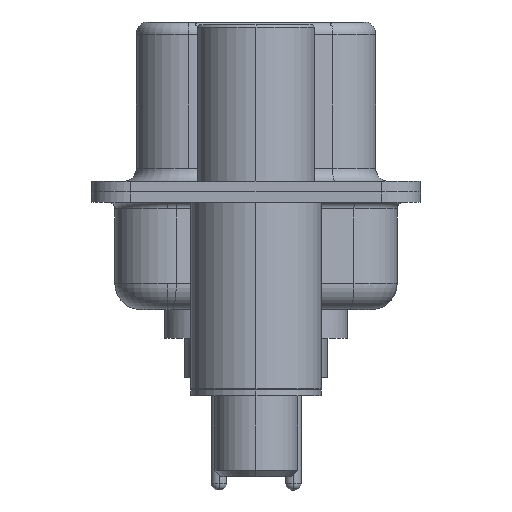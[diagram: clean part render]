
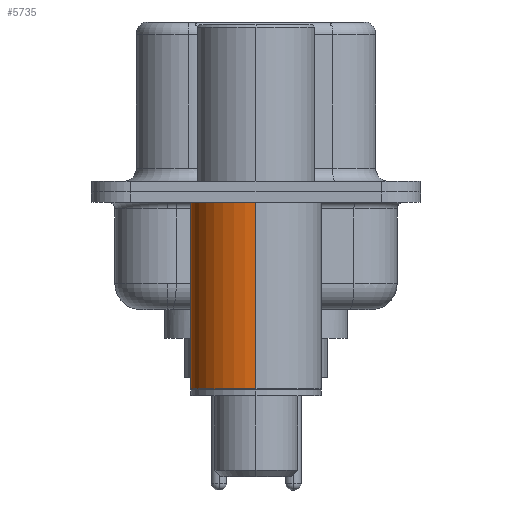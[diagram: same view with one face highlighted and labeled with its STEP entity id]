
A CAD part, left-side view. The second image highlights one B-rep face of the part: STEP entity #5735.
In plain terms, the highlighted cylindrical face has radius 2.5 mm (diameter 5 mm), a partial arc.
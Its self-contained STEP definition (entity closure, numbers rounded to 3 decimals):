
#570 = ORIENTED_EDGE ( 'NONE', *, *, #3838, .F. ) ;
#767 = CARTESIAN_POINT ( 'NONE',  ( 0., 0., -7.525 ) ) ;
#917 = EDGE_LOOP ( 'NONE', ( #12664, #6063, #570, #17866 ) ) ;
#1201 = AXIS2_PLACEMENT_3D ( 'NONE', #21291, #8077, #12361 ) ;
#1298 = VERTEX_POINT ( 'NONE', #20996 ) ;
#2603 = VECTOR ( 'NONE', #26259, 1000. ) ;
#3025 = DIRECTION ( 'NONE',  ( 1., 0., 0. ) ) ;
#3763 = CYLINDRICAL_SURFACE ( 'NONE', #17589, 2.5 ) ;
#3836 = VERTEX_POINT ( 'NONE', #18754 ) ;
#3838 = EDGE_CURVE ( 'NONE', #1298, #3836, #13167, .T. ) ;
#5735 = ADVANCED_FACE ( 'NONE', ( #10599 ), #3763, .T. ) ;
#6063 = ORIENTED_EDGE ( 'NONE', *, *, #20919, .T. ) ;
#8077 = DIRECTION ( 'NONE',  ( 0., 0., 1. ) ) ;
#9319 = VERTEX_POINT ( 'NONE', #25199 ) ;
#10195 = CARTESIAN_POINT ( 'NONE',  ( 2.5, 0., 0.581 ) ) ;
#10599 = FACE_OUTER_BOUND ( 'NONE', #917, .T. ) ;
#12361 = DIRECTION ( 'NONE',  ( 1., 0., 0. ) ) ;
#12529 = CIRCLE ( 'NONE', #14786, 2.5 ) ;
#12664 = ORIENTED_EDGE ( 'NONE', *, *, #16217, .T. ) ;
#13167 = CIRCLE ( 'NONE', #1201, 2.5 ) ;
#13356 = LINE ( 'NONE', #14674, #24122 ) ;
#13838 = CARTESIAN_POINT ( 'NONE',  ( 0., 0., 0.581 ) ) ;
#14674 = CARTESIAN_POINT ( 'NONE',  ( -2.5, 0., 0.581 ) ) ;
#14786 = AXIS2_PLACEMENT_3D ( 'NONE', #767, #16775, #3025 ) ;
#16217 = EDGE_CURVE ( 'NONE', #9319, #25919, #12529, .T. ) ;
#16775 = DIRECTION ( 'NONE',  ( 0., 0., 1. ) ) ;
#17589 = AXIS2_PLACEMENT_3D ( 'NONE', #13838, #27592, #20643 ) ;
#17866 = ORIENTED_EDGE ( 'NONE', *, *, #27214, .F. ) ;
#18754 = CARTESIAN_POINT ( 'NONE',  ( -2.5, 0., -0.4 ) ) ;
#20643 = DIRECTION ( 'NONE',  ( 1., 0., 0. ) ) ;
#20919 = EDGE_CURVE ( 'NONE', #25919, #3836, #13356, .T. ) ;
#20920 = LINE ( 'NONE', #10195, #2603 ) ;
#20996 = CARTESIAN_POINT ( 'NONE',  ( 2.5, 0., -0.4 ) ) ;
#21291 = CARTESIAN_POINT ( 'NONE',  ( 0., 0., -0.4 ) ) ;
#21585 = DIRECTION ( 'NONE',  ( 0., 0., 1. ) ) ;
#24122 = VECTOR ( 'NONE', #21585, 1000. ) ;
#25199 = CARTESIAN_POINT ( 'NONE',  ( 2.5, 0., -7.525 ) ) ;
#25919 = VERTEX_POINT ( 'NONE', #28984 ) ;
#26259 = DIRECTION ( 'NONE',  ( 0., 0., 1. ) ) ;
#27214 = EDGE_CURVE ( 'NONE', #9319, #1298, #20920, .T. ) ;
#27592 = DIRECTION ( 'NONE',  ( 0., 0., 1. ) ) ;
#28984 = CARTESIAN_POINT ( 'NONE',  ( -2.5, 0., -7.525 ) ) ;
